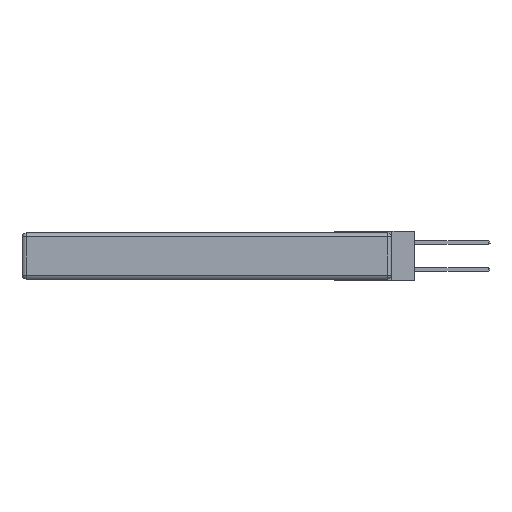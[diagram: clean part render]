
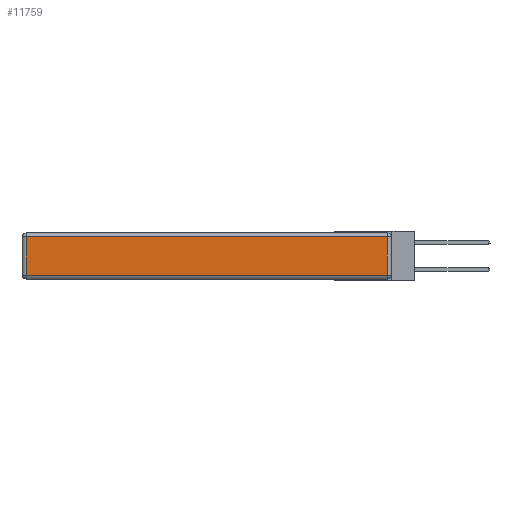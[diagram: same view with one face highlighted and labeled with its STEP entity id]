
A CAD part, left-side view. The second image highlights one B-rep face of the part: STEP entity #11759.
In plain terms, the highlighted planar face has unit normal (-1, 0, 0).
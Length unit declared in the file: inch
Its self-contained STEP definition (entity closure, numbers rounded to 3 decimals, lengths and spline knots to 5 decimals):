
#284 = DIRECTION ( 'NONE',  ( 0., 0., 1. ) ) ;
#373 = LINE ( 'NONE', #10357, #8407 ) ;
#762 = ORIENTED_EDGE ( 'NONE', *, *, #14180, .T. ) ;
#1391 = DIRECTION ( 'NONE',  ( -1., 0., 0. ) ) ;
#2064 = AXIS2_PLACEMENT_3D ( 'NONE', #8218, #1391, #284 ) ;
#2243 = CARTESIAN_POINT ( 'NONE',  ( 0., 0.03, -0.313 ) ) ;
#2868 = DIRECTION ( 'NONE',  ( 0., 0., -1. ) ) ;
#2943 = CARTESIAN_POINT ( 'NONE',  ( 0., 2.72, -0.03 ) ) ;
#4223 = FACE_OUTER_BOUND ( 'NONE', #12163, .T. ) ;
#5111 = EDGE_CURVE ( 'NONE', #13707, #13971, #6608, .T. ) ;
#5554 = DIRECTION ( 'NONE',  ( 0., 1., 0. ) ) ;
#6608 = LINE ( 'NONE', #8266, #9090 ) ;
#7090 = ORIENTED_EDGE ( 'NONE', *, *, #12589, .T. ) ;
#7189 = PLANE ( 'NONE',  #2064 ) ;
#7934 = ORIENTED_EDGE ( 'NONE', *, *, #10806, .T. ) ;
#8202 = CARTESIAN_POINT ( 'NONE',  ( 0., 0., -0.313 ) ) ;
#8218 = CARTESIAN_POINT ( 'NONE',  ( 0., 0., -0.343 ) ) ;
#8266 = CARTESIAN_POINT ( 'NONE',  ( 0., 0.03, -0.343 ) ) ;
#8407 = VECTOR ( 'NONE', #5554, 39.37008 ) ;
#8620 = ORIENTED_EDGE ( 'NONE', *, *, #5111, .T. ) ;
#8678 = VECTOR ( 'NONE', #2868, 39.37008 ) ;
#9032 = VERTEX_POINT ( 'NONE', #13036 ) ;
#9090 = VECTOR ( 'NONE', #14014, 39.37008 ) ;
#9247 = VERTEX_POINT ( 'NONE', #2943 ) ;
#10100 = LINE ( 'NONE', #12017, #8678 ) ;
#10245 = LINE ( 'NONE', #8202, #10946 ) ;
#10357 = CARTESIAN_POINT ( 'NONE',  ( 0., 2.75, -0.03 ) ) ;
#10806 = EDGE_CURVE ( 'NONE', #9247, #9032, #10100, .T. ) ;
#10946 = VECTOR ( 'NONE', #13944, 39.37008 ) ;
#11759 = ADVANCED_FACE ( 'NONE', ( #4223 ), #7189, .T. ) ;
#12011 = CARTESIAN_POINT ( 'NONE',  ( 0., 0.03, -0.03 ) ) ;
#12017 = CARTESIAN_POINT ( 'NONE',  ( 0., 2.72, -0.343 ) ) ;
#12163 = EDGE_LOOP ( 'NONE', ( #7090, #8620, #762, #7934 ) ) ;
#12589 = EDGE_CURVE ( 'NONE', #9032, #13707, #10245, .T. ) ;
#13036 = CARTESIAN_POINT ( 'NONE',  ( 0., 2.72, -0.313 ) ) ;
#13707 = VERTEX_POINT ( 'NONE', #2243 ) ;
#13944 = DIRECTION ( 'NONE',  ( 0., -1., 0. ) ) ;
#13971 = VERTEX_POINT ( 'NONE', #12011 ) ;
#14014 = DIRECTION ( 'NONE',  ( 0., 0., 1. ) ) ;
#14180 = EDGE_CURVE ( 'NONE', #13971, #9247, #373, .T. ) ;
